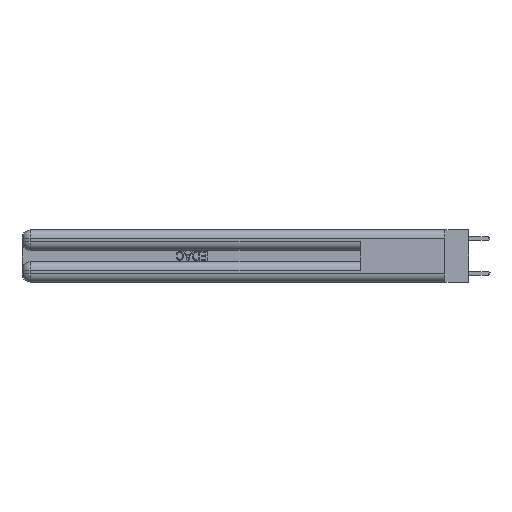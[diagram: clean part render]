
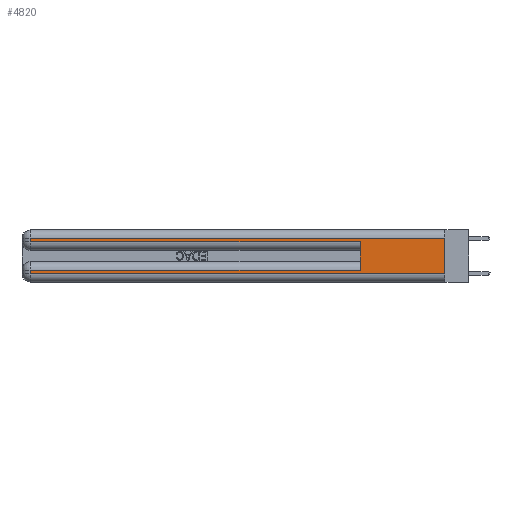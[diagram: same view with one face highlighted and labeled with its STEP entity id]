
A CAD part, left-side view. The second image highlights one B-rep face of the part: STEP entity #4820.
In plain terms, the highlighted planar face has unit normal (-1, 0, 0).
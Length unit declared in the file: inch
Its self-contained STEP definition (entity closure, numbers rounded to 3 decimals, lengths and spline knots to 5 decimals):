
#42 = LINE ( 'NONE', #9599, #8004 ) ;
#212 = ORIENTED_EDGE ( 'NONE', *, *, #17458, .T. ) ;
#959 = ORIENTED_EDGE ( 'NONE', *, *, #3437, .T. ) ;
#1783 = VECTOR ( 'NONE', #17500, 39.37008 ) ;
#3239 = VERTEX_POINT ( 'NONE', #11316 ) ;
#3437 = EDGE_CURVE ( 'NONE', #25839, #34129, #18523, .T. ) ;
#3825 = LINE ( 'NONE', #17349, #31247 ) ;
#4478 = VERTEX_POINT ( 'NONE', #32759 ) ;
#4793 = ORIENTED_EDGE ( 'NONE', *, *, #5752, .F. ) ;
#4820 = ADVANCED_FACE ( 'NONE', ( #10996 ), #7631, .F. ) ;
#5752 = EDGE_CURVE ( 'NONE', #3239, #34129, #3825, .T. ) ;
#6056 = EDGE_CURVE ( 'NONE', #10514, #25839, #31631, .T. ) ;
#7151 = AXIS2_PLACEMENT_3D ( 'NONE', #26199, #12975, #31493 ) ;
#7243 = VECTOR ( 'NONE', #21384, 39.37008 ) ;
#7325 = LINE ( 'NONE', #9278, #13560 ) ;
#7631 = PLANE ( 'NONE',  #7151 ) ;
#8004 = VECTOR ( 'NONE', #12301, 39.37008 ) ;
#8074 = VECTOR ( 'NONE', #32353, 39.37008 ) ;
#9278 = CARTESIAN_POINT ( 'NONE',  ( 0., 0., 0.31 ) ) ;
#9381 = DIRECTION ( 'NONE',  ( 0., 0., 1. ) ) ;
#9414 = CARTESIAN_POINT ( 'NONE',  ( 0., 0., 0.285 ) ) ;
#9599 = CARTESIAN_POINT ( 'NONE',  ( 0., 0., 0.06 ) ) ;
#9759 = EDGE_CURVE ( 'NONE', #18936, #10514, #7325, .T. ) ;
#10514 = VERTEX_POINT ( 'NONE', #12380 ) ;
#10996 = FACE_OUTER_BOUND ( 'NONE', #26146, .T. ) ;
#11316 = CARTESIAN_POINT ( 'NONE',  ( 0., 0.6, 0.085 ) ) ;
#12301 = DIRECTION ( 'NONE',  ( 0., -1., 0. ) ) ;
#12380 = CARTESIAN_POINT ( 'NONE',  ( 0., 2.94, 0.31 ) ) ;
#12511 = VERTEX_POINT ( 'NONE', #27140 ) ;
#12975 = DIRECTION ( 'NONE',  ( 1., 0., 0. ) ) ;
#13560 = VECTOR ( 'NONE', #30494, 39.37008 ) ;
#14178 = ORIENTED_EDGE ( 'NONE', *, *, #20798, .T. ) ;
#17349 = CARTESIAN_POINT ( 'NONE',  ( 0., 0.6, 0.145 ) ) ;
#17458 = EDGE_CURVE ( 'NONE', #12511, #29016, #26984, .T. ) ;
#17500 = DIRECTION ( 'NONE',  ( 0., -1., 0. ) ) ;
#17516 = CARTESIAN_POINT ( 'NONE',  ( 0., 2.94, 0.37 ) ) ;
#17611 = VECTOR ( 'NONE', #20223, 39.37008 ) ;
#18394 = ORIENTED_EDGE ( 'NONE', *, *, #9759, .T. ) ;
#18439 = CARTESIAN_POINT ( 'NONE',  ( 0., 0.6, 0.285 ) ) ;
#18523 = LINE ( 'NONE', #9414, #1783 ) ;
#18936 = VERTEX_POINT ( 'NONE', #32231 ) ;
#19572 = CARTESIAN_POINT ( 'NONE',  ( 0., 2.94, 0.06 ) ) ;
#20022 = VECTOR ( 'NONE', #28054, 39.37008 ) ;
#20169 = CARTESIAN_POINT ( 'NONE',  ( 0., 2.94, 0.37 ) ) ;
#20223 = DIRECTION ( 'NONE',  ( 0., 0., -1. ) ) ;
#20798 = EDGE_CURVE ( 'NONE', #3239, #12511, #21463, .T. ) ;
#21384 = DIRECTION ( 'NONE',  ( 0., 1., 0. ) ) ;
#21463 = LINE ( 'NONE', #29256, #7243 ) ;
#22276 = LINE ( 'NONE', #27081, #8074 ) ;
#22595 = ORIENTED_EDGE ( 'NONE', *, *, #6056, .T. ) ;
#24163 = ORIENTED_EDGE ( 'NONE', *, *, #33649, .F. ) ;
#25109 = CARTESIAN_POINT ( 'NONE',  ( 0., 2.94, 0.285 ) ) ;
#25839 = VERTEX_POINT ( 'NONE', #25109 ) ;
#25901 = EDGE_CURVE ( 'NONE', #29016, #4478, #42, .T. ) ;
#26146 = EDGE_LOOP ( 'NONE', ( #24163, #18394, #22595, #959, #4793, #14178, #212, #30987 ) ) ;
#26199 = CARTESIAN_POINT ( 'NONE',  ( 0., 0., 0.37 ) ) ;
#26984 = LINE ( 'NONE', #20169, #20022 ) ;
#27081 = CARTESIAN_POINT ( 'NONE',  ( 0., 0., 0.37 ) ) ;
#27140 = CARTESIAN_POINT ( 'NONE',  ( 0., 2.94, 0.085 ) ) ;
#28054 = DIRECTION ( 'NONE',  ( 0., 0., -1. ) ) ;
#29016 = VERTEX_POINT ( 'NONE', #19572 ) ;
#29256 = CARTESIAN_POINT ( 'NONE',  ( 0., 0., 0.085 ) ) ;
#30494 = DIRECTION ( 'NONE',  ( 0., 1., 0. ) ) ;
#30987 = ORIENTED_EDGE ( 'NONE', *, *, #25901, .T. ) ;
#31247 = VECTOR ( 'NONE', #9381, 39.37008 ) ;
#31493 = DIRECTION ( 'NONE',  ( 0., 0., -1. ) ) ;
#31631 = LINE ( 'NONE', #17516, #17611 ) ;
#32231 = CARTESIAN_POINT ( 'NONE',  ( 0., 0., 0.31 ) ) ;
#32353 = DIRECTION ( 'NONE',  ( 0., 0., -1. ) ) ;
#32759 = CARTESIAN_POINT ( 'NONE',  ( 0., 0., 0.06 ) ) ;
#33649 = EDGE_CURVE ( 'NONE', #18936, #4478, #22276, .T. ) ;
#34129 = VERTEX_POINT ( 'NONE', #18439 ) ;
